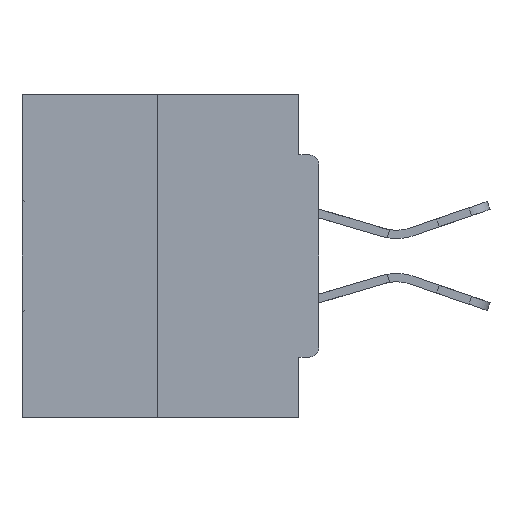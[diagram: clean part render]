
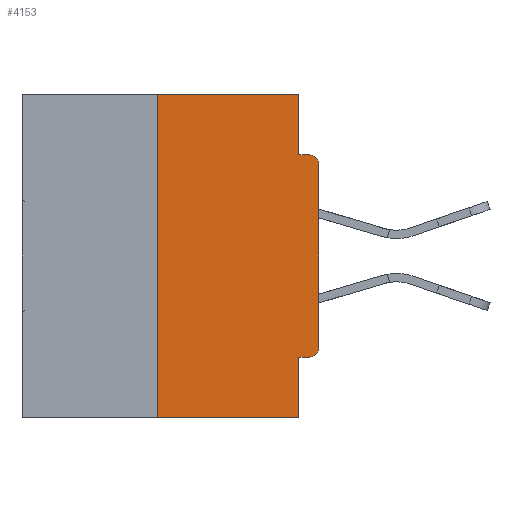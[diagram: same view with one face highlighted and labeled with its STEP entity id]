
A CAD part, left-side view. The second image highlights one B-rep face of the part: STEP entity #4153.
In plain terms, the highlighted planar face has unit normal (-1, 0, 0).
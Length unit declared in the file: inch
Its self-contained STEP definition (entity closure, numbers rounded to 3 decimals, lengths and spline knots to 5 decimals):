
#137 = DIRECTION ( 'NONE',  ( 0., 0., -1. ) ) ;
#227 = CARTESIAN_POINT ( 'NONE',  ( 0., 0.25, 0. ) ) ;
#714 = CARTESIAN_POINT ( 'NONE',  ( 0., 0.25, -0.5 ) ) ;
#1324 = VECTOR ( 'NONE', #15149, 39.37008 ) ;
#1651 = ORIENTED_EDGE ( 'NONE', *, *, #39903, .T. ) ;
#2025 = CARTESIAN_POINT ( 'NONE',  ( 0., 0.46, -0.5 ) ) ;
#3046 = VERTEX_POINT ( 'NONE', #24994 ) ;
#3249 = CARTESIAN_POINT ( 'NONE',  ( 0., 0.015, -0.1085 ) ) ;
#3311 = LINE ( 'NONE', #36840, #8437 ) ;
#3578 = ORIENTED_EDGE ( 'NONE', *, *, #32217, .F. ) ;
#3941 = DIRECTION ( 'NONE',  ( 0., -1., 0. ) ) ;
#4153 = ADVANCED_FACE ( 'NONE', ( #17649 ), #6060, .F. ) ;
#4250 = LINE ( 'NONE', #30667, #37844 ) ;
#4517 = ORIENTED_EDGE ( 'NONE', *, *, #32597, .F. ) ;
#5238 = CARTESIAN_POINT ( 'NONE',  ( 0., 0.031, -0.5 ) ) ;
#5492 = CARTESIAN_POINT ( 'NONE',  ( 0., 0., -0.1085 ) ) ;
#6060 = PLANE ( 'NONE',  #8909 ) ;
#6395 = DIRECTION ( 'NONE',  ( -1., 0., 0. ) ) ;
#6938 = ORIENTED_EDGE ( 'NONE', *, *, #21463, .F. ) ;
#7681 = VERTEX_POINT ( 'NONE', #714 ) ;
#7800 = VERTEX_POINT ( 'NONE', #5238 ) ;
#8437 = VECTOR ( 'NONE', #40304, 39.37008 ) ;
#8775 = EDGE_LOOP ( 'NONE', ( #17914, #6938, #14359, #11916, #4517, #34044, #1651, #16808, #28684, #3578 ) ) ;
#8909 = AXIS2_PLACEMENT_3D ( 'NONE', #35676, #12619, #38507 ) ;
#9349 = VECTOR ( 'NONE', #9498, 39.37008 ) ;
#9498 = DIRECTION ( 'NONE',  ( 0., 0., 1. ) ) ;
#9740 = VERTEX_POINT ( 'NONE', #16358 ) ;
#9876 = VERTEX_POINT ( 'NONE', #28543 ) ;
#10537 = VECTOR ( 'NONE', #137, 39.37008 ) ;
#11904 = DIRECTION ( 'NONE',  ( 0., 0., -1. ) ) ;
#11916 = ORIENTED_EDGE ( 'NONE', *, *, #20998, .F. ) ;
#12353 = VERTEX_POINT ( 'NONE', #37383 ) ;
#12529 = LINE ( 'NONE', #38842, #10537 ) ;
#12619 = DIRECTION ( 'NONE',  ( 1., 0., 0. ) ) ;
#12830 = DIRECTION ( 'NONE',  ( 0., 0., -1. ) ) ;
#13081 = LINE ( 'NONE', #22385, #20723 ) ;
#13760 = CARTESIAN_POINT ( 'NONE',  ( 0., 0.015, -0.4065 ) ) ;
#14359 = ORIENTED_EDGE ( 'NONE', *, *, #19754, .T. ) ;
#15132 = CIRCLE ( 'NONE', #19785, 0.015 ) ;
#15149 = DIRECTION ( 'NONE',  ( 0., -1., 0. ) ) ;
#15166 = CARTESIAN_POINT ( 'NONE',  ( 0., 0., -0.3915 ) ) ;
#15490 = AXIS2_PLACEMENT_3D ( 'NONE', #3249, #6395, #12830 ) ;
#16358 = CARTESIAN_POINT ( 'NONE',  ( 0., 0.015, -0.0935 ) ) ;
#16808 = ORIENTED_EDGE ( 'NONE', *, *, #26176, .T. ) ;
#17649 = FACE_OUTER_BOUND ( 'NONE', #8775, .T. ) ;
#17914 = ORIENTED_EDGE ( 'NONE', *, *, #42100, .F. ) ;
#18019 = LINE ( 'NONE', #227, #9349 ) ;
#19657 = VECTOR ( 'NONE', #3941, 39.37008 ) ;
#19754 = EDGE_CURVE ( 'NONE', #7681, #7800, #21244, .T. ) ;
#19785 = AXIS2_PLACEMENT_3D ( 'NONE', #41081, #38163, #11904 ) ;
#20723 = VECTOR ( 'NONE', #29810, 39.37008 ) ;
#20998 = EDGE_CURVE ( 'NONE', #12353, #7800, #4250, .T. ) ;
#21160 = LINE ( 'NONE', #39543, #19657 ) ;
#21244 = LINE ( 'NONE', #2025, #1324 ) ;
#21463 = EDGE_CURVE ( 'NONE', #7681, #27134, #18019, .T. ) ;
#22385 = CARTESIAN_POINT ( 'NONE',  ( 0., 0., 0. ) ) ;
#23484 = LINE ( 'NONE', #33533, #32616 ) ;
#24994 = CARTESIAN_POINT ( 'NONE',  ( 0., 0.031, 0. ) ) ;
#26176 = EDGE_CURVE ( 'NONE', #34049, #9740, #41160, .T. ) ;
#27134 = VERTEX_POINT ( 'NONE', #41724 ) ;
#27353 = EDGE_CURVE ( 'NONE', #9876, #9740, #21160, .T. ) ;
#28543 = CARTESIAN_POINT ( 'NONE',  ( 0., 0.031, -0.0935 ) ) ;
#28684 = ORIENTED_EDGE ( 'NONE', *, *, #27353, .F. ) ;
#29810 = DIRECTION ( 'NONE',  ( 0., 0., 1. ) ) ;
#30519 = DIRECTION ( 'NONE',  ( 0., -1., 0. ) ) ;
#30667 = CARTESIAN_POINT ( 'NONE',  ( 0., 0.031, -0.5 ) ) ;
#31464 = EDGE_CURVE ( 'NONE', #40432, #40747, #15132, .T. ) ;
#32217 = EDGE_CURVE ( 'NONE', #3046, #9876, #12529, .T. ) ;
#32597 = EDGE_CURVE ( 'NONE', #40432, #12353, #3311, .T. ) ;
#32616 = VECTOR ( 'NONE', #30519, 39.37008 ) ;
#33533 = CARTESIAN_POINT ( 'NONE',  ( 0., 0.46, 0. ) ) ;
#34044 = ORIENTED_EDGE ( 'NONE', *, *, #31464, .T. ) ;
#34049 = VERTEX_POINT ( 'NONE', #5492 ) ;
#35676 = CARTESIAN_POINT ( 'NONE',  ( 0., 0.46, 0. ) ) ;
#36840 = CARTESIAN_POINT ( 'NONE',  ( 0., 0., -0.4065 ) ) ;
#37383 = CARTESIAN_POINT ( 'NONE',  ( 0., 0.031, -0.4065 ) ) ;
#37844 = VECTOR ( 'NONE', #40527, 39.37008 ) ;
#38163 = DIRECTION ( 'NONE',  ( -1., 0., 0. ) ) ;
#38507 = DIRECTION ( 'NONE',  ( 0., 0., -1. ) ) ;
#38842 = CARTESIAN_POINT ( 'NONE',  ( 0., 0.031, 0. ) ) ;
#39543 = CARTESIAN_POINT ( 'NONE',  ( 0., 0., -0.0935 ) ) ;
#39903 = EDGE_CURVE ( 'NONE', #40747, #34049, #13081, .T. ) ;
#40304 = DIRECTION ( 'NONE',  ( 0., 1., 0. ) ) ;
#40432 = VERTEX_POINT ( 'NONE', #13760 ) ;
#40527 = DIRECTION ( 'NONE',  ( 0., 0., -1. ) ) ;
#40747 = VERTEX_POINT ( 'NONE', #15166 ) ;
#41081 = CARTESIAN_POINT ( 'NONE',  ( 0., 0.015, -0.3915 ) ) ;
#41160 = CIRCLE ( 'NONE', #15490, 0.015 ) ;
#41724 = CARTESIAN_POINT ( 'NONE',  ( 0., 0.25, 0. ) ) ;
#42100 = EDGE_CURVE ( 'NONE', #27134, #3046, #23484, .T. ) ;
